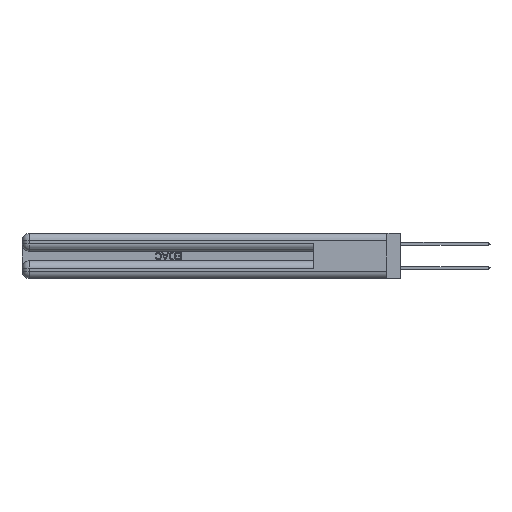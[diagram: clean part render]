
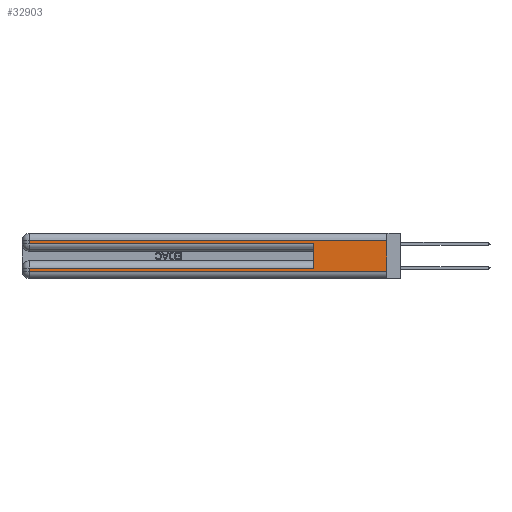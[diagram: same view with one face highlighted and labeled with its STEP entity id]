
A CAD part, left-side view. The second image highlights one B-rep face of the part: STEP entity #32903.
In plain terms, the highlighted planar face has unit normal (-1, 0, 0).
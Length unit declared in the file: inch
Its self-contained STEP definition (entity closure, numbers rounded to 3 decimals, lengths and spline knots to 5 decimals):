
#676 = VERTEX_POINT ( 'NONE', #16637 ) ;
#799 = ORIENTED_EDGE ( 'NONE', *, *, #49929, .F. ) ;
#2400 = LINE ( 'NONE', #42983, #12892 ) ;
#2630 = EDGE_CURVE ( 'NONE', #34136, #9691, #42601, .T. ) ;
#4282 = CARTESIAN_POINT ( 'NONE',  ( 0., 2.94, 0.37 ) ) ;
#4834 = LINE ( 'NONE', #32482, #34889 ) ;
#4945 = CARTESIAN_POINT ( 'NONE',  ( 0., 0., 0.37 ) ) ;
#6255 = EDGE_LOOP ( 'NONE', ( #23546, #15591, #6302, #20500, #799, #44766, #25409, #18723 ) ) ;
#6302 = ORIENTED_EDGE ( 'NONE', *, *, #32812, .T. ) ;
#8042 = AXIS2_PLACEMENT_3D ( 'NONE', #4945, #32382, #8918 ) ;
#8695 = VERTEX_POINT ( 'NONE', #39286 ) ;
#8804 = LINE ( 'NONE', #45118, #19324 ) ;
#8918 = DIRECTION ( 'NONE',  ( 0., 0., -1. ) ) ;
#8958 = EDGE_CURVE ( 'NONE', #32055, #23650, #8804, .T. ) ;
#9691 = VERTEX_POINT ( 'NONE', #25794 ) ;
#10837 = EDGE_CURVE ( 'NONE', #32055, #676, #28260, .T. ) ;
#12892 = VECTOR ( 'NONE', #19786, 39.37008 ) ;
#13849 = LINE ( 'NONE', #40777, #43628 ) ;
#14645 = VERTEX_POINT ( 'NONE', #45472 ) ;
#15591 = ORIENTED_EDGE ( 'NONE', *, *, #10837, .T. ) ;
#15605 = DIRECTION ( 'NONE',  ( 0., -1., 0. ) ) ;
#16637 = CARTESIAN_POINT ( 'NONE',  ( 0., 2.94, 0.31 ) ) ;
#17555 = EDGE_CURVE ( 'NONE', #9691, #23650, #2400, .T. ) ;
#18723 = ORIENTED_EDGE ( 'NONE', *, *, #17555, .T. ) ;
#19324 = VECTOR ( 'NONE', #21918, 39.37008 ) ;
#19786 = DIRECTION ( 'NONE',  ( 0., -1., 0. ) ) ;
#19850 = DIRECTION ( 'NONE',  ( 0., 0., -1. ) ) ;
#20479 = CARTESIAN_POINT ( 'NONE',  ( 0., 0., 0.31 ) ) ;
#20500 = ORIENTED_EDGE ( 'NONE', *, *, #29249, .T. ) ;
#21918 = DIRECTION ( 'NONE',  ( 0., 0., -1. ) ) ;
#23227 = VECTOR ( 'NONE', #19850, 39.37008 ) ;
#23546 = ORIENTED_EDGE ( 'NONE', *, *, #8958, .F. ) ;
#23650 = VERTEX_POINT ( 'NONE', #37485 ) ;
#23904 = DIRECTION ( 'NONE',  ( 0., 0., -1. ) ) ;
#24335 = DIRECTION ( 'NONE',  ( 0., 0., 1. ) ) ;
#24397 = DIRECTION ( 'NONE',  ( 0., 1., 0. ) ) ;
#25409 = ORIENTED_EDGE ( 'NONE', *, *, #2630, .T. ) ;
#25794 = CARTESIAN_POINT ( 'NONE',  ( 0., 2.94, 0.06 ) ) ;
#27042 = VECTOR ( 'NONE', #24397, 39.37008 ) ;
#27377 = CARTESIAN_POINT ( 'NONE',  ( 0., 0., 0.31 ) ) ;
#28083 = CARTESIAN_POINT ( 'NONE',  ( 0., 0.6, 0.145 ) ) ;
#28260 = LINE ( 'NONE', #20479, #27042 ) ;
#29249 = EDGE_CURVE ( 'NONE', #48741, #14645, #4834, .T. ) ;
#32055 = VERTEX_POINT ( 'NONE', #27377 ) ;
#32382 = DIRECTION ( 'NONE',  ( 1., 0., 0. ) ) ;
#32482 = CARTESIAN_POINT ( 'NONE',  ( 0., 0., 0.285 ) ) ;
#32800 = VECTOR ( 'NONE', #24335, 39.37008 ) ;
#32812 = EDGE_CURVE ( 'NONE', #676, #48741, #48889, .T. ) ;
#32903 = ADVANCED_FACE ( 'NONE', ( #41651 ), #47729, .F. ) ;
#34136 = VERTEX_POINT ( 'NONE', #42439 ) ;
#34889 = VECTOR ( 'NONE', #15605, 39.37008 ) ;
#37485 = CARTESIAN_POINT ( 'NONE',  ( 0., 0., 0.06 ) ) ;
#37712 = EDGE_CURVE ( 'NONE', #8695, #34136, #13849, .T. ) ;
#39286 = CARTESIAN_POINT ( 'NONE',  ( 0., 0.6, 0.085 ) ) ;
#40552 = CARTESIAN_POINT ( 'NONE',  ( 0., 2.94, 0.285 ) ) ;
#40777 = CARTESIAN_POINT ( 'NONE',  ( 0., 0., 0.085 ) ) ;
#41651 = FACE_OUTER_BOUND ( 'NONE', #6255, .T. ) ;
#42439 = CARTESIAN_POINT ( 'NONE',  ( 0., 2.94, 0.085 ) ) ;
#42601 = LINE ( 'NONE', #46941, #23227 ) ;
#42983 = CARTESIAN_POINT ( 'NONE',  ( 0., 0., 0.06 ) ) ;
#43061 = LINE ( 'NONE', #28083, #32800 ) ;
#43628 = VECTOR ( 'NONE', #44663, 39.37008 ) ;
#44663 = DIRECTION ( 'NONE',  ( 0., 1., 0. ) ) ;
#44766 = ORIENTED_EDGE ( 'NONE', *, *, #37712, .T. ) ;
#45118 = CARTESIAN_POINT ( 'NONE',  ( 0., 0., 0.37 ) ) ;
#45472 = CARTESIAN_POINT ( 'NONE',  ( 0., 0.6, 0.285 ) ) ;
#46941 = CARTESIAN_POINT ( 'NONE',  ( 0., 2.94, 0.37 ) ) ;
#47676 = VECTOR ( 'NONE', #23904, 39.37008 ) ;
#47729 = PLANE ( 'NONE',  #8042 ) ;
#48741 = VERTEX_POINT ( 'NONE', #40552 ) ;
#48889 = LINE ( 'NONE', #4282, #47676 ) ;
#49929 = EDGE_CURVE ( 'NONE', #8695, #14645, #43061, .T. ) ;
